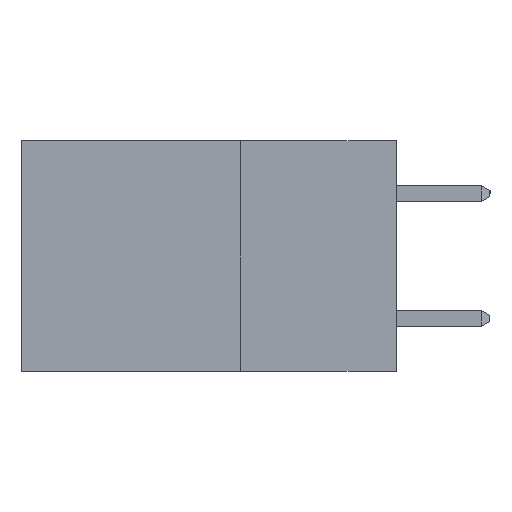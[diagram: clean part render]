
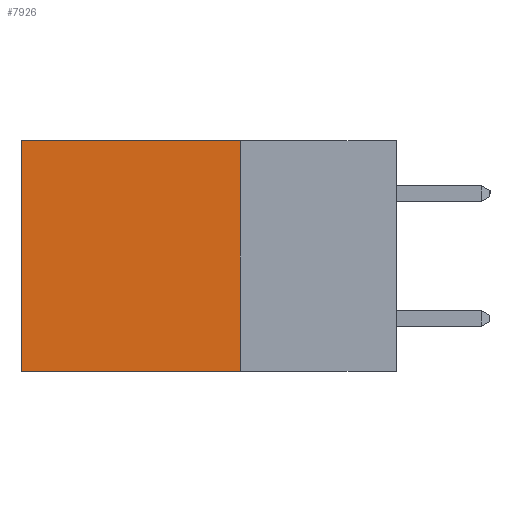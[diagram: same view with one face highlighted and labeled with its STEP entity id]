
A CAD part, left-side view. The second image highlights one B-rep face of the part: STEP entity #7926.
In plain terms, the highlighted planar face has unit normal (-1, 0, 0).
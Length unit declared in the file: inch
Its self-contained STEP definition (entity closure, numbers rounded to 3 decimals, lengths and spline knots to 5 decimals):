
#44 = EDGE_LOOP ( 'NONE', ( #10453, #9341, #482, #243 ) ) ;
#243 = ORIENTED_EDGE ( 'NONE', *, *, #7693, .T. ) ;
#289 = DIRECTION ( 'NONE',  ( 1., 0., 0. ) ) ;
#482 = ORIENTED_EDGE ( 'NONE', *, *, #9484, .F. ) ;
#1223 = EDGE_CURVE ( 'NONE', #7801, #3044, #1791, .T. ) ;
#1731 = CARTESIAN_POINT ( 'NONE',  ( 0.2615, 0.25, 0. ) ) ;
#1791 = LINE ( 'NONE', #2788, #4932 ) ;
#2053 = CARTESIAN_POINT ( 'NONE',  ( 0.2615, 0.25, -0.37 ) ) ;
#2201 = CARTESIAN_POINT ( 'NONE',  ( 0.2615, 0.6, -0.37 ) ) ;
#2788 = CARTESIAN_POINT ( 'NONE',  ( 0.2615, 0.25, -0.37 ) ) ;
#2797 = VECTOR ( 'NONE', #8436, 39.37008 ) ;
#3044 = VERTEX_POINT ( 'NONE', #2201 ) ;
#3799 = CARTESIAN_POINT ( 'NONE',  ( 0.2615, 0.25, -0.37 ) ) ;
#4190 = DIRECTION ( 'NONE',  ( 0., 1., 0. ) ) ;
#4317 = DIRECTION ( 'NONE',  ( 0., 0., -1. ) ) ;
#4596 = LINE ( 'NONE', #3799, #8646 ) ;
#4692 = VECTOR ( 'NONE', #4823, 39.37008 ) ;
#4748 = EDGE_CURVE ( 'NONE', #9089, #3044, #6144, .T. ) ;
#4823 = DIRECTION ( 'NONE',  ( 0., 1., 0. ) ) ;
#4932 = VECTOR ( 'NONE', #4190, 39.37008 ) ;
#5524 = CARTESIAN_POINT ( 'NONE',  ( 0.2615, 0.6, 0. ) ) ;
#5555 = VERTEX_POINT ( 'NONE', #1731 ) ;
#6144 = LINE ( 'NONE', #10047, #2797 ) ;
#6442 = CARTESIAN_POINT ( 'NONE',  ( 0.2615, 0.25, 0. ) ) ;
#6656 = CARTESIAN_POINT ( 'NONE',  ( 0.2615, 0.25, -0.37 ) ) ;
#7087 = DIRECTION ( 'NONE',  ( 0., 0., -1. ) ) ;
#7195 = AXIS2_PLACEMENT_3D ( 'NONE', #2053, #289, #4317 ) ;
#7693 = EDGE_CURVE ( 'NONE', #5555, #9089, #8288, .T. ) ;
#7801 = VERTEX_POINT ( 'NONE', #6656 ) ;
#7926 = ADVANCED_FACE ( 'NONE', ( #10203 ), #9414, .F. ) ;
#8288 = LINE ( 'NONE', #6442, #4692 ) ;
#8436 = DIRECTION ( 'NONE',  ( 0., 0., -1. ) ) ;
#8646 = VECTOR ( 'NONE', #7087, 39.37008 ) ;
#9089 = VERTEX_POINT ( 'NONE', #5524 ) ;
#9341 = ORIENTED_EDGE ( 'NONE', *, *, #1223, .F. ) ;
#9414 = PLANE ( 'NONE',  #7195 ) ;
#9484 = EDGE_CURVE ( 'NONE', #5555, #7801, #4596, .T. ) ;
#10047 = CARTESIAN_POINT ( 'NONE',  ( 0.2615, 0.6, -0.37 ) ) ;
#10203 = FACE_OUTER_BOUND ( 'NONE', #44, .T. ) ;
#10453 = ORIENTED_EDGE ( 'NONE', *, *, #4748, .T. ) ;
